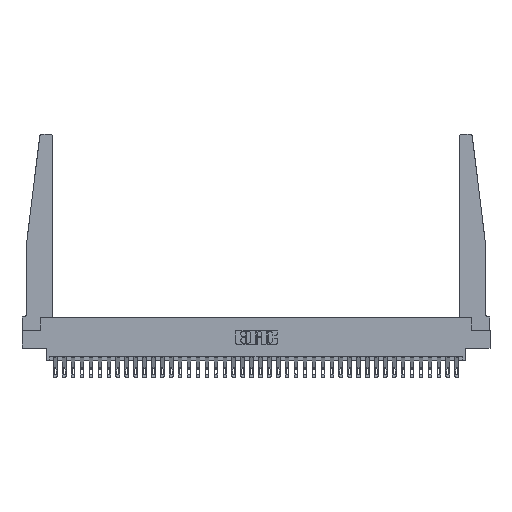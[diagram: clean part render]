
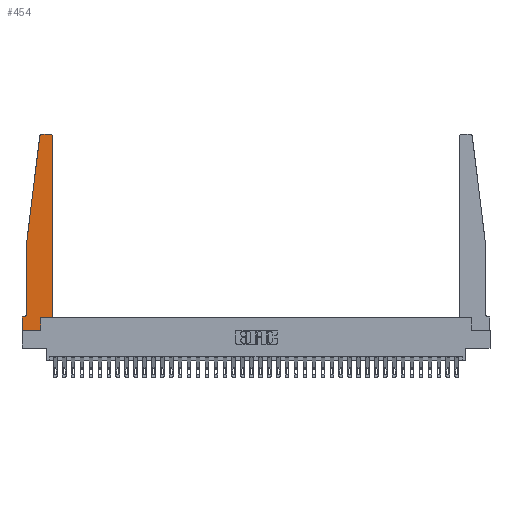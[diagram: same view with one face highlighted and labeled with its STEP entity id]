
A CAD part, top view. The second image highlights one B-rep face of the part: STEP entity #454.
In plain terms, the highlighted planar face has unit normal (0, 0, 1).
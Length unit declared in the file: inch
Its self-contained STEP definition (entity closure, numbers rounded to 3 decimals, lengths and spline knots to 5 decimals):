
#454 = ADVANCED_FACE ( 'NONE', ( #12277 ), #10842, .T. ) ;
#892 = CARTESIAN_POINT ( 'NONE',  ( 0.425, 0.18, 0.37 ) ) ;
#1958 = DIRECTION ( 'NONE',  ( 1., 0., 0. ) ) ;
#2314 = DIRECTION ( 'NONE',  ( 1., 0., 0. ) ) ;
#2801 = DIRECTION ( 'NONE',  ( 0., -1., 0. ) ) ;
#3108 = DIRECTION ( 'NONE',  ( -0.122, -0.992, 0. ) ) ;
#3216 = LINE ( 'NONE', #20740, #18334 ) ;
#3678 = ORIENTED_EDGE ( 'NONE', *, *, #25232, .T. ) ;
#3859 = CIRCLE ( 'NONE', #17386, 0.03 ) ;
#3991 = LINE ( 'NONE', #892, #24530 ) ;
#4636 = DIRECTION ( 'NONE',  ( 1., 0., 0. ) ) ;
#5213 = CARTESIAN_POINT ( 'NONE',  ( 0.27653, 2.72, 0.37 ) ) ;
#5370 = ORIENTED_EDGE ( 'NONE', *, *, #32956, .T. ) ;
#5686 = CARTESIAN_POINT ( 'NONE',  ( 0., 0., 0.37 ) ) ;
#5791 = CIRCLE ( 'NONE', #9591, 0.05 ) ;
#6554 = VERTEX_POINT ( 'NONE', #6599 ) ;
#6599 = CARTESIAN_POINT ( 'NONE',  ( 0., 0., 0.37 ) ) ;
#6619 = VERTEX_POINT ( 'NONE', #22865 ) ;
#7453 = ORIENTED_EDGE ( 'NONE', *, *, #17394, .T. ) ;
#7920 = DIRECTION ( 'NONE',  ( 1., 0., 0. ) ) ;
#8245 = DIRECTION ( 'NONE',  ( 1., 0., 0. ) ) ;
#8380 = LINE ( 'NONE', #5686, #10063 ) ;
#8639 = VERTEX_POINT ( 'NONE', #19851 ) ;
#9135 = CARTESIAN_POINT ( 'NONE',  ( 0.2605, 0.18, 0.37 ) ) ;
#9591 = AXIS2_PLACEMENT_3D ( 'NONE', #31992, #15966, #34667 ) ;
#9990 = VERTEX_POINT ( 'NONE', #14128 ) ;
#10063 = VECTOR ( 'NONE', #27102, 39.37008 ) ;
#10362 = CARTESIAN_POINT ( 'NONE',  ( 0.425, 2.72, 0.37 ) ) ;
#10842 = PLANE ( 'NONE',  #18573 ) ;
#11194 = VERTEX_POINT ( 'NONE', #21445 ) ;
#12277 = FACE_OUTER_BOUND ( 'NONE', #29375, .T. ) ;
#12514 = ORIENTED_EDGE ( 'NONE', *, *, #19735, .T. ) ;
#12932 = ORIENTED_EDGE ( 'NONE', *, *, #21563, .T. ) ;
#12984 = LINE ( 'NONE', #16182, #21755 ) ;
#14128 = CARTESIAN_POINT ( 'NONE',  ( 0.2605, 0.18, 0.37 ) ) ;
#14137 = VERTEX_POINT ( 'NONE', #33191 ) ;
#14532 = DIRECTION ( 'NONE',  ( 0., 1., 0. ) ) ;
#14595 = ORIENTED_EDGE ( 'NONE', *, *, #24148, .T. ) ;
#14643 = VERTEX_POINT ( 'NONE', #24387 ) ;
#15104 = CARTESIAN_POINT ( 'NONE',  ( 0.25, 2.75, 0.37 ) ) ;
#15966 = DIRECTION ( 'NONE',  ( 0., 0., -1. ) ) ;
#15998 = AXIS2_PLACEMENT_3D ( 'NONE', #34383, #18401, #2314 ) ;
#16099 = DIRECTION ( 'NONE',  ( -1., 0., 0. ) ) ;
#16182 = CARTESIAN_POINT ( 'NONE',  ( 0.065, 1.25, 0.37 ) ) ;
#16255 = ORIENTED_EDGE ( 'NONE', *, *, #23492, .T. ) ;
#16314 = VECTOR ( 'NONE', #31121, 39.37008 ) ;
#16703 = VECTOR ( 'NONE', #3108, 39.37008 ) ;
#17094 = EDGE_CURVE ( 'NONE', #8639, #9990, #19695, .T. ) ;
#17362 = VERTEX_POINT ( 'NONE', #29803 ) ;
#17386 = AXIS2_PLACEMENT_3D ( 'NONE', #5213, #23939, #7920 ) ;
#17394 = EDGE_CURVE ( 'NONE', #14137, #17362, #30929, .T. ) ;
#17933 = ORIENTED_EDGE ( 'NONE', *, *, #17094, .T. ) ;
#18334 = VECTOR ( 'NONE', #1958, 39.37008 ) ;
#18401 = DIRECTION ( 'NONE',  ( 0., 0., 1. ) ) ;
#18573 = AXIS2_PLACEMENT_3D ( 'NONE', #21605, #24278, #8245 ) ;
#19695 = LINE ( 'NONE', #9135, #25102 ) ;
#19735 = EDGE_CURVE ( 'NONE', #6619, #24616, #3991, .T. ) ;
#19851 = CARTESIAN_POINT ( 'NONE',  ( 0.2605, 0., 0.37 ) ) ;
#20312 = CARTESIAN_POINT ( 'NONE',  ( 0.065, 0.2375, 0.37 ) ) ;
#20693 = CARTESIAN_POINT ( 'NONE',  ( 0.425, 0.18, 0.37 ) ) ;
#20740 = CARTESIAN_POINT ( 'NONE',  ( 0., 0., 0.37 ) ) ;
#21397 = CARTESIAN_POINT ( 'NONE',  ( 0.065, 0.1875, 0.37 ) ) ;
#21445 = CARTESIAN_POINT ( 'NONE',  ( 0.395, 2.75, 0.37 ) ) ;
#21563 = EDGE_CURVE ( 'NONE', #29196, #14137, #3859, .T. ) ;
#21605 = CARTESIAN_POINT ( 'NONE',  ( 0., 0.1875, 0.37 ) ) ;
#21755 = VECTOR ( 'NONE', #2801, 39.37008 ) ;
#22865 = CARTESIAN_POINT ( 'NONE',  ( 0.425, 0.18, 0.37 ) ) ;
#23368 = ORIENTED_EDGE ( 'NONE', *, *, #23585, .T. ) ;
#23492 = EDGE_CURVE ( 'NONE', #14643, #32654, #32249, .T. ) ;
#23585 = EDGE_CURVE ( 'NONE', #32654, #6554, #8380, .T. ) ;
#23823 = VERTEX_POINT ( 'NONE', #20312 ) ;
#23939 = DIRECTION ( 'NONE',  ( 0., 0., 1. ) ) ;
#24147 = LINE ( 'NONE', #20693, #31252 ) ;
#24148 = EDGE_CURVE ( 'NONE', #17362, #23823, #12984, .T. ) ;
#24278 = DIRECTION ( 'NONE',  ( 0., 0., 1. ) ) ;
#24387 = CARTESIAN_POINT ( 'NONE',  ( 0.015, 0.1875, 0.37 ) ) ;
#24530 = VECTOR ( 'NONE', #25076, 39.37008 ) ;
#24548 = CARTESIAN_POINT ( 'NONE',  ( 0.065, 1.25, 0.37 ) ) ;
#24616 = VERTEX_POINT ( 'NONE', #10362 ) ;
#24671 = EDGE_CURVE ( 'NONE', #23823, #14643, #5791, .T. ) ;
#24903 = CIRCLE ( 'NONE', #15998, 0.03 ) ;
#25076 = DIRECTION ( 'NONE',  ( 0., 1., 0. ) ) ;
#25102 = VECTOR ( 'NONE', #14532, 39.37008 ) ;
#25232 = EDGE_CURVE ( 'NONE', #6554, #8639, #3216, .T. ) ;
#27102 = DIRECTION ( 'NONE',  ( 0., -1., 0. ) ) ;
#28819 = ORIENTED_EDGE ( 'NONE', *, *, #24671, .T. ) ;
#29196 = VERTEX_POINT ( 'NONE', #34066 ) ;
#29375 = EDGE_LOOP ( 'NONE', ( #33404, #12932, #7453, #14595, #28819, #16255, #23368, #3678, #17933, #5370, #12514, #34671 ) ) ;
#29803 = CARTESIAN_POINT ( 'NONE',  ( 0.065, 1.25, 0.37 ) ) ;
#30343 = EDGE_CURVE ( 'NONE', #11194, #29196, #30549, .T. ) ;
#30549 = LINE ( 'NONE', #15104, #16314 ) ;
#30929 = LINE ( 'NONE', #24548, #16703 ) ;
#31121 = DIRECTION ( 'NONE',  ( -1., 0., 0. ) ) ;
#31252 = VECTOR ( 'NONE', #4636, 39.37008 ) ;
#31401 = VECTOR ( 'NONE', #16099, 39.37008 ) ;
#31992 = CARTESIAN_POINT ( 'NONE',  ( 0.015, 0.2375, 0.37 ) ) ;
#32249 = LINE ( 'NONE', #21397, #31401 ) ;
#32654 = VERTEX_POINT ( 'NONE', #32872 ) ;
#32872 = CARTESIAN_POINT ( 'NONE',  ( 0., 0.1875, 0.37 ) ) ;
#32956 = EDGE_CURVE ( 'NONE', #9990, #6619, #24147, .T. ) ;
#33191 = CARTESIAN_POINT ( 'NONE',  ( 0.24675, 2.72367, 0.37 ) ) ;
#33404 = ORIENTED_EDGE ( 'NONE', *, *, #30343, .T. ) ;
#34066 = CARTESIAN_POINT ( 'NONE',  ( 0.27653, 2.75, 0.37 ) ) ;
#34269 = EDGE_CURVE ( 'NONE', #24616, #11194, #24903, .T. ) ;
#34383 = CARTESIAN_POINT ( 'NONE',  ( 0.395, 2.72, 0.37 ) ) ;
#34667 = DIRECTION ( 'NONE',  ( -1., 0., 0. ) ) ;
#34671 = ORIENTED_EDGE ( 'NONE', *, *, #34269, .T. ) ;
